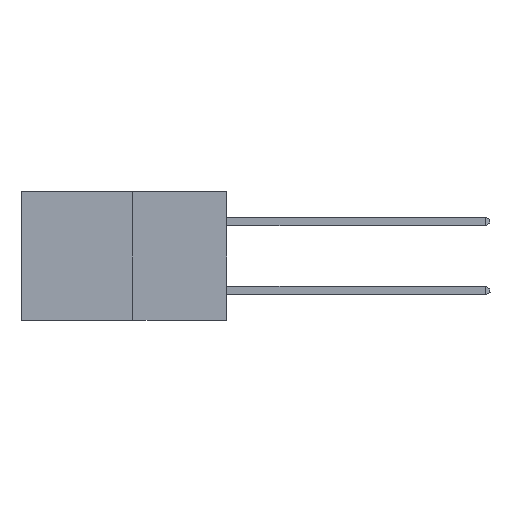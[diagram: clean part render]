
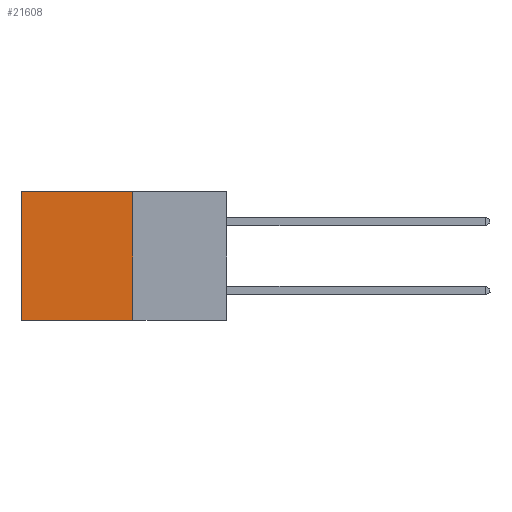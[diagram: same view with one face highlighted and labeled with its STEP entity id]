
A CAD part, left-side view. The second image highlights one B-rep face of the part: STEP entity #21608.
In plain terms, the highlighted planar face has unit normal (-1, 0, 0).
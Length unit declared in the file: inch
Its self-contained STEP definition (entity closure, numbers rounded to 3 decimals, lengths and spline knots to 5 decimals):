
#260 = VERTEX_POINT ( 'NONE', #17697 ) ;
#566 = VECTOR ( 'NONE', #21449, 39.37008 ) ;
#1424 = ORIENTED_EDGE ( 'NONE', *, *, #7561, .F. ) ;
#1760 = ORIENTED_EDGE ( 'NONE', *, *, #21348, .F. ) ;
#2118 = DIRECTION ( 'NONE',  ( 0., 1., 0. ) ) ;
#2591 = CARTESIAN_POINT ( 'NONE',  ( 0.277, 0.27, -0.37 ) ) ;
#2614 = CARTESIAN_POINT ( 'NONE',  ( 0.277, 0.27, -0.37 ) ) ;
#3312 = VECTOR ( 'NONE', #15033, 39.37008 ) ;
#3472 = ORIENTED_EDGE ( 'NONE', *, *, #12091, .T. ) ;
#3666 = LINE ( 'NONE', #10492, #11698 ) ;
#4326 = DIRECTION ( 'NONE',  ( 0., 0., -1. ) ) ;
#4434 = VERTEX_POINT ( 'NONE', #13353 ) ;
#4963 = VERTEX_POINT ( 'NONE', #14643 ) ;
#5338 = DIRECTION ( 'NONE',  ( 0., 0., -1. ) ) ;
#7561 = EDGE_CURVE ( 'NONE', #4434, #4963, #14284, .T. ) ;
#8334 = EDGE_CURVE ( 'NONE', #18370, #4963, #17523, .T. ) ;
#8562 = ORIENTED_EDGE ( 'NONE', *, *, #8334, .T. ) ;
#9252 = CARTESIAN_POINT ( 'NONE',  ( 0.277, 0.59, 0. ) ) ;
#10420 = EDGE_LOOP ( 'NONE', ( #8562, #1424, #1760, #3472 ) ) ;
#10492 = CARTESIAN_POINT ( 'NONE',  ( 0.277, 0.27, -0.37 ) ) ;
#11000 = AXIS2_PLACEMENT_3D ( 'NONE', #2614, #14546, #4326 ) ;
#11423 = FACE_OUTER_BOUND ( 'NONE', #10420, .T. ) ;
#11698 = VECTOR ( 'NONE', #5338, 39.37008 ) ;
#12091 = EDGE_CURVE ( 'NONE', #260, #18370, #21877, .T. ) ;
#12365 = CARTESIAN_POINT ( 'NONE',  ( 0.277, 0.27, 0. ) ) ;
#13353 = CARTESIAN_POINT ( 'NONE',  ( 0.277, 0.27, -0.37 ) ) ;
#13846 = VECTOR ( 'NONE', #2118, 39.37008 ) ;
#14284 = LINE ( 'NONE', #2591, #566 ) ;
#14546 = DIRECTION ( 'NONE',  ( 1., 0., 0. ) ) ;
#14643 = CARTESIAN_POINT ( 'NONE',  ( 0.277, 0.59, -0.37 ) ) ;
#15033 = DIRECTION ( 'NONE',  ( 0., 0., -1. ) ) ;
#17523 = LINE ( 'NONE', #20217, #3312 ) ;
#17697 = CARTESIAN_POINT ( 'NONE',  ( 0.277, 0.27, 0. ) ) ;
#18370 = VERTEX_POINT ( 'NONE', #9252 ) ;
#20217 = CARTESIAN_POINT ( 'NONE',  ( 0.277, 0.59, -0.37 ) ) ;
#21348 = EDGE_CURVE ( 'NONE', #260, #4434, #3666, .T. ) ;
#21402 = PLANE ( 'NONE',  #11000 ) ;
#21449 = DIRECTION ( 'NONE',  ( 0., 1., 0. ) ) ;
#21608 = ADVANCED_FACE ( 'NONE', ( #11423 ), #21402, .F. ) ;
#21877 = LINE ( 'NONE', #12365, #13846 ) ;
